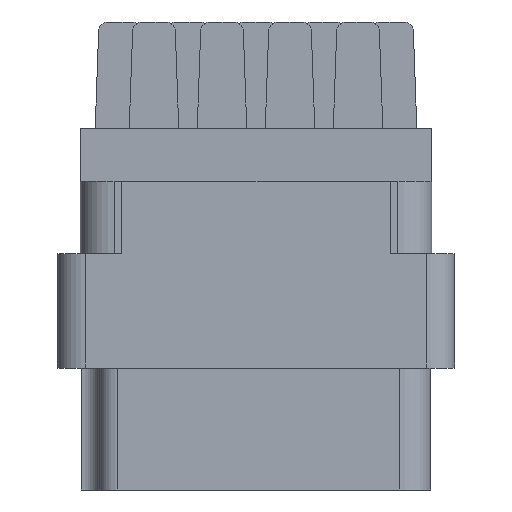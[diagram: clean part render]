
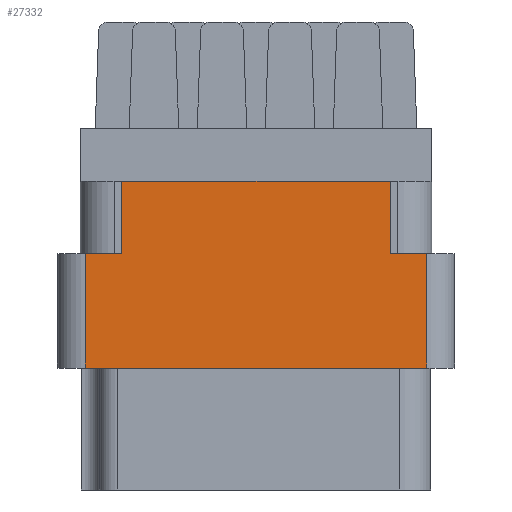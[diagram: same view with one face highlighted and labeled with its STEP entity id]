
A CAD part, left-side view. The second image highlights one B-rep face of the part: STEP entity #27332.
In plain terms, the highlighted planar face has unit normal (-1, 0, 0).
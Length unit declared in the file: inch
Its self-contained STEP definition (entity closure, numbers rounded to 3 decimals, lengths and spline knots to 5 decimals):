
#151 = CARTESIAN_POINT ( 'NONE',  ( -1.296, -0.296, -0.117 ) ) ;
#208 = CARTESIAN_POINT ( 'NONE',  ( -1.296, -0.296, -0.277 ) ) ;
#1291 = VERTEX_POINT ( 'NONE', #10415 ) ;
#1950 = LINE ( 'NONE', #37522, #5413 ) ;
#2287 = CARTESIAN_POINT ( 'NONE',  ( -1.296, -0.376, -0.529 ) ) ;
#2416 = DIRECTION ( 'NONE',  ( 0., -1., 0. ) ) ;
#2717 = EDGE_LOOP ( 'NONE', ( #27881, #13180, #14351, #14308, #4122, #37059, #9406, #9028 ) ) ;
#2825 = CARTESIAN_POINT ( 'NONE',  ( -1.296, 0.376, -0.798 ) ) ;
#2881 = CARTESIAN_POINT ( 'NONE',  ( -1.296, 0., -0.277 ) ) ;
#3062 = CARTESIAN_POINT ( 'NONE',  ( -1.296, -0.438, -0.798 ) ) ;
#4122 = ORIENTED_EDGE ( 'NONE', *, *, #19507, .F. ) ;
#4894 = VERTEX_POINT ( 'NONE', #151 ) ;
#5413 = VECTOR ( 'NONE', #30135, 39.37008 ) ;
#5733 = CARTESIAN_POINT ( 'NONE',  ( -1.296, -0.296, -0.277 ) ) ;
#5790 = VECTOR ( 'NONE', #10128, 39.37008 ) ;
#6519 = LINE ( 'NONE', #10589, #5790 ) ;
#6629 = LINE ( 'NONE', #2825, #23284 ) ;
#7183 = EDGE_CURVE ( 'NONE', #42089, #12881, #14435, .T. ) ;
#7618 = VECTOR ( 'NONE', #18837, 39.37008 ) ;
#8118 = VERTEX_POINT ( 'NONE', #208 ) ;
#8470 = VERTEX_POINT ( 'NONE', #31931 ) ;
#9028 = ORIENTED_EDGE ( 'NONE', *, *, #47126, .F. ) ;
#9406 = ORIENTED_EDGE ( 'NONE', *, *, #10463, .F. ) ;
#9813 = VECTOR ( 'NONE', #20566, 39.37008 ) ;
#10128 = DIRECTION ( 'NONE',  ( 0., 0., 1. ) ) ;
#10415 = CARTESIAN_POINT ( 'NONE',  ( -1.296, 0.376, -0.529 ) ) ;
#10463 = EDGE_CURVE ( 'NONE', #8470, #4894, #15714, .T. ) ;
#10589 = CARTESIAN_POINT ( 'NONE',  ( -1.296, -0.376, -0.798 ) ) ;
#11611 = CARTESIAN_POINT ( 'NONE',  ( -1.296, 0.296, -0.277 ) ) ;
#12759 = DIRECTION ( 'NONE',  ( 0., 0., 1. ) ) ;
#12881 = VERTEX_POINT ( 'NONE', #13936 ) ;
#12930 = LINE ( 'NONE', #2881, #46875 ) ;
#13180 = ORIENTED_EDGE ( 'NONE', *, *, #41703, .T. ) ;
#13936 = CARTESIAN_POINT ( 'NONE',  ( -1.296, 0.296, -0.277 ) ) ;
#14308 = ORIENTED_EDGE ( 'NONE', *, *, #20309, .T. ) ;
#14351 = ORIENTED_EDGE ( 'NONE', *, *, #32574, .F. ) ;
#14435 = LINE ( 'NONE', #20892, #17685 ) ;
#15714 = LINE ( 'NONE', #26451, #7618 ) ;
#17685 = VECTOR ( 'NONE', #28993, 39.37008 ) ;
#18837 = DIRECTION ( 'NONE',  ( 0., -1., 0. ) ) ;
#19507 = EDGE_CURVE ( 'NONE', #8118, #20697, #12930, .T. ) ;
#20309 = EDGE_CURVE ( 'NONE', #39083, #20697, #6519, .T. ) ;
#20566 = DIRECTION ( 'NONE',  ( 0., 0., 1. ) ) ;
#20697 = VERTEX_POINT ( 'NONE', #46317 ) ;
#20892 = CARTESIAN_POINT ( 'NONE',  ( -1.296, 0., -0.277 ) ) ;
#21231 = FACE_OUTER_BOUND ( 'NONE', #2717, .T. ) ;
#23284 = VECTOR ( 'NONE', #39102, 39.37008 ) ;
#25197 = VECTOR ( 'NONE', #29051, 39.37008 ) ;
#26451 = CARTESIAN_POINT ( 'NONE',  ( -1.296, 0.438, -0.117 ) ) ;
#27332 = ADVANCED_FACE ( 'NONE', ( #21231 ), #35769, .T. ) ;
#27881 = ORIENTED_EDGE ( 'NONE', *, *, #7183, .F. ) ;
#28993 = DIRECTION ( 'NONE',  ( 0., -1., 0. ) ) ;
#29051 = DIRECTION ( 'NONE',  ( 0., 0., 1. ) ) ;
#30135 = DIRECTION ( 'NONE',  ( 0., 1., 0. ) ) ;
#31190 = CARTESIAN_POINT ( 'NONE',  ( -1.296, 0.376, -0.277 ) ) ;
#31931 = CARTESIAN_POINT ( 'NONE',  ( -1.296, 0.296, -0.117 ) ) ;
#32574 = EDGE_CURVE ( 'NONE', #39083, #1291, #1950, .T. ) ;
#35769 = PLANE ( 'NONE',  #36726 ) ;
#36671 = LINE ( 'NONE', #11611, #25197 ) ;
#36726 = AXIS2_PLACEMENT_3D ( 'NONE', #3062, #43624, #12759 ) ;
#37059 = ORIENTED_EDGE ( 'NONE', *, *, #45098, .T. ) ;
#37522 = CARTESIAN_POINT ( 'NONE',  ( -1.296, 0., -0.529 ) ) ;
#39083 = VERTEX_POINT ( 'NONE', #2287 ) ;
#39102 = DIRECTION ( 'NONE',  ( 0., 0., -1. ) ) ;
#41703 = EDGE_CURVE ( 'NONE', #42089, #1291, #6629, .T. ) ;
#42089 = VERTEX_POINT ( 'NONE', #31190 ) ;
#43624 = DIRECTION ( 'NONE',  ( -1., 0., 0. ) ) ;
#45098 = EDGE_CURVE ( 'NONE', #8118, #4894, #45344, .T. ) ;
#45344 = LINE ( 'NONE', #5733, #9813 ) ;
#46317 = CARTESIAN_POINT ( 'NONE',  ( -1.296, -0.376, -0.277 ) ) ;
#46875 = VECTOR ( 'NONE', #2416, 39.37008 ) ;
#47126 = EDGE_CURVE ( 'NONE', #12881, #8470, #36671, .T. ) ;
